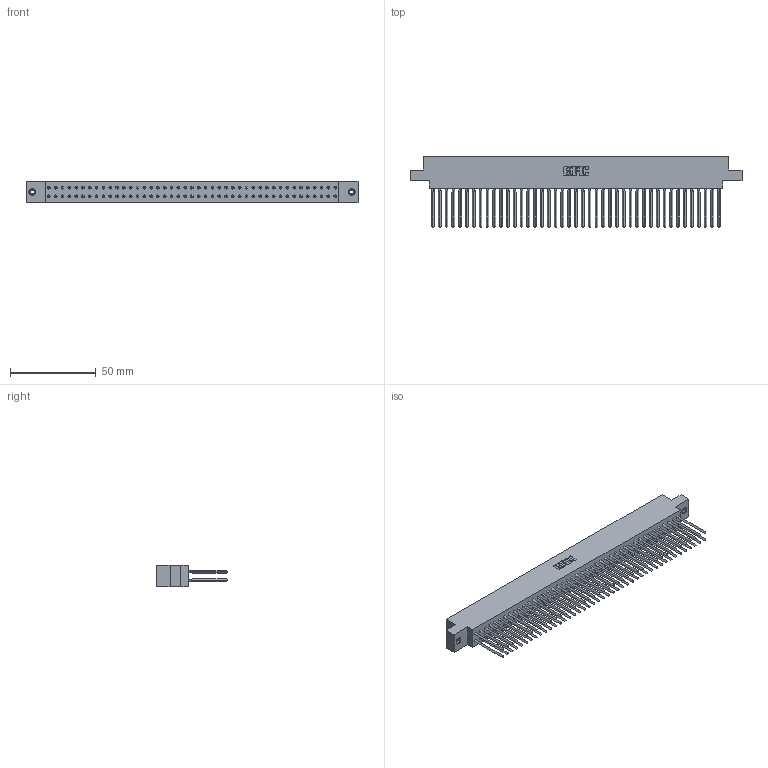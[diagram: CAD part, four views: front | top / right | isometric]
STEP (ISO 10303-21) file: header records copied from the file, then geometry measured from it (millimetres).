
FILE_DESCRIPTION (( 'STEP AP203' ), '1' );
FILE_NAME ('317-086-543-808.STEP', '2020-02-28T10:49:39', ( '' ), ( '' ), 'SwSTEP 2.0', 'SolidWorks 2016', '' );
FILE_SCHEMA (( 'CONFIG_CONTROL_DESIGN' ));
Length unit declared in the file: inch
Products named in the file (4): 317 Part_.156 Dia - TI; 345-250-001_345-250-003-102; 317-086-543-808; 317-290-001_543
Assembly tree (89 placements, depth 2):
  317-086-543-808
    317 Part_.156 Dia - TI
    317-290-001_543  x86
    345-250-001_345-250-003-102  x2
Bounding box: 193.09 x 41.15 x 12.7 mm (x, y, z)
Volume: 32861.9 mm3; surface area: 49914.2 mm2
Topology: 89 solids, 89 shells, 7816 faces, 21653 edges, 13940 vertices
Faces by surface type: plane 6368, cylinder 1088, bspline 344, cone 12, torus 4
Entity records: 63203 total; most frequent: CARTESIAN_POINT 11414, ORIENTED_EDGE 10906, DIRECTION 9137, EDGE_CURVE 5453, LINE 5177, VECTOR 5177, VERTEX_POINT 3625, AXIS2_PLACEMENT_3D 1980
